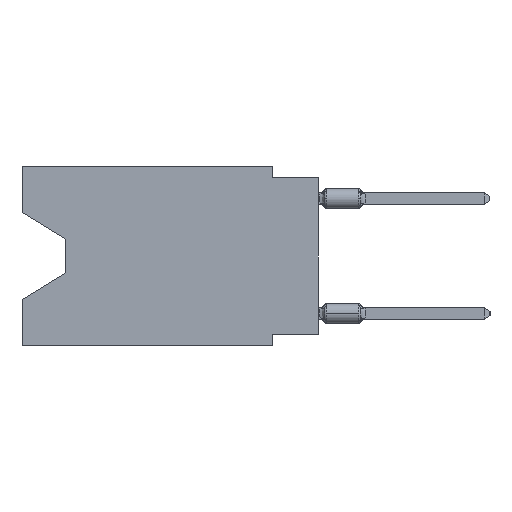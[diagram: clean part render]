
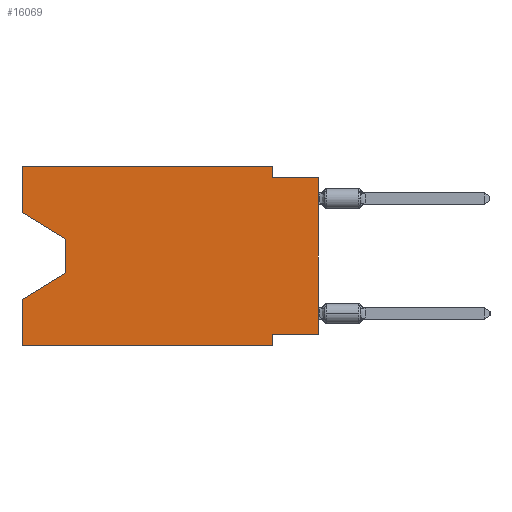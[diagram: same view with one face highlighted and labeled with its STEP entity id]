
A CAD part, left-side view. The second image highlights one B-rep face of the part: STEP entity #16069.
In plain terms, the highlighted planar face has unit normal (-1, 0, 0).
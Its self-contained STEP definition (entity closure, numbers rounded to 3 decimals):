
#253 = DIRECTION ( 'NONE',  ( 0., -0.855, -0.519 ) ) ;
#407 = VECTOR ( 'NONE', #17483, 1000. ) ;
#1360 = CARTESIAN_POINT ( 'NONE',  ( 0., 0., -9.271 ) ) ;
#1849 = LINE ( 'NONE', #1360, #12850 ) ;
#1931 = LINE ( 'NONE', #11982, #15742 ) ;
#2307 = LINE ( 'NONE', #31834, #407 ) ;
#2446 = EDGE_CURVE ( 'NONE', #3500, #23172, #26357, .T. ) ;
#2697 = ORIENTED_EDGE ( 'NONE', *, *, #17128, .T. ) ;
#2833 = ORIENTED_EDGE ( 'NONE', *, *, #22995, .F. ) ;
#3056 = CARTESIAN_POINT ( 'NONE',  ( 0., 16.383, -2.546 ) ) ;
#3317 = VECTOR ( 'NONE', #18878, 1000. ) ;
#3348 = EDGE_CURVE ( 'NONE', #29747, #30917, #1849, .T. ) ;
#3500 = VERTEX_POINT ( 'NONE', #32190 ) ;
#4700 = ORIENTED_EDGE ( 'NONE', *, *, #19175, .F. ) ;
#5203 = CARTESIAN_POINT ( 'NONE',  ( 0., 16.383, -9.906 ) ) ;
#6359 = VERTEX_POINT ( 'NONE', #16911 ) ;
#6776 = CARTESIAN_POINT ( 'NONE',  ( 0., 2.54, -9.271 ) ) ;
#7807 = LINE ( 'NONE', #28116, #12186 ) ;
#7935 = VECTOR ( 'NONE', #253, 1000. ) ;
#8007 = VERTEX_POINT ( 'NONE', #12410 ) ;
#8150 = LINE ( 'NONE', #10787, #27226 ) ;
#8793 = CARTESIAN_POINT ( 'NONE',  ( 0., 13.97, -5.893 ) ) ;
#9356 = VERTEX_POINT ( 'NONE', #8793 ) ;
#9927 = CARTESIAN_POINT ( 'NONE',  ( 0., 2.54, -9.906 ) ) ;
#10622 = EDGE_CURVE ( 'NONE', #30917, #29506, #10952, .T. ) ;
#10629 = LINE ( 'NONE', #3056, #7935 ) ;
#10787 = CARTESIAN_POINT ( 'NONE',  ( 0., 16.383, 0. ) ) ;
#10952 = LINE ( 'NONE', #31084, #3317 ) ;
#11600 = ORIENTED_EDGE ( 'NONE', *, *, #25312, .T. ) ;
#11870 = ORIENTED_EDGE ( 'NONE', *, *, #10622, .F. ) ;
#11897 = DIRECTION ( 'NONE',  ( 0., 1., 0. ) ) ;
#11982 = CARTESIAN_POINT ( 'NONE',  ( 0., 13.97, -5.893 ) ) ;
#12186 = VECTOR ( 'NONE', #30104, 1000. ) ;
#12410 = CARTESIAN_POINT ( 'NONE',  ( 0., 16.383, -2.546 ) ) ;
#12850 = VECTOR ( 'NONE', #11897, 1000. ) ;
#13371 = ORIENTED_EDGE ( 'NONE', *, *, #19501, .T. ) ;
#13765 = VECTOR ( 'NONE', #29118, 1000. ) ;
#13810 = CARTESIAN_POINT ( 'NONE',  ( 0., 16.383, 0. ) ) ;
#14072 = AXIS2_PLACEMENT_3D ( 'NONE', #29518, #21774, #19460 ) ;
#14195 = CARTESIAN_POINT ( 'NONE',  ( 0., 0., -9.271 ) ) ;
#14386 = LINE ( 'NONE', #31880, #29523 ) ;
#14493 = FACE_OUTER_BOUND ( 'NONE', #32248, .T. ) ;
#15328 = ORIENTED_EDGE ( 'NONE', *, *, #3348, .F. ) ;
#15532 = EDGE_CURVE ( 'NONE', #20619, #28723, #8150, .T. ) ;
#15742 = VECTOR ( 'NONE', #22058, 1000. ) ;
#15854 = ORIENTED_EDGE ( 'NONE', *, *, #15532, .F. ) ;
#16069 = ADVANCED_FACE ( 'NONE', ( #14493 ), #27216, .F. ) ;
#16404 = EDGE_CURVE ( 'NONE', #23172, #27235, #29970, .T. ) ;
#16911 = CARTESIAN_POINT ( 'NONE',  ( 0., 0., -0.635 ) ) ;
#17128 = EDGE_CURVE ( 'NONE', #20619, #29506, #18854, .T. ) ;
#17483 = DIRECTION ( 'NONE',  ( 0., 0., 1. ) ) ;
#18854 = LINE ( 'NONE', #28923, #22419 ) ;
#18878 = DIRECTION ( 'NONE',  ( 0., 0., -1. ) ) ;
#19046 = LINE ( 'NONE', #21842, #13765 ) ;
#19081 = VECTOR ( 'NONE', #28669, 1000. ) ;
#19175 = EDGE_CURVE ( 'NONE', #27235, #6359, #7807, .T. ) ;
#19460 = DIRECTION ( 'NONE',  ( 0., 0., -1. ) ) ;
#19501 = EDGE_CURVE ( 'NONE', #28805, #9356, #14386, .T. ) ;
#20581 = EDGE_CURVE ( 'NONE', #8007, #28805, #10629, .T. ) ;
#20619 = VERTEX_POINT ( 'NONE', #5203 ) ;
#20765 = EDGE_CURVE ( 'NONE', #29747, #6359, #19046, .T. ) ;
#21084 = CARTESIAN_POINT ( 'NONE',  ( 0., 2.54, 0. ) ) ;
#21774 = DIRECTION ( 'NONE',  ( 1., 0., 0. ) ) ;
#21842 = CARTESIAN_POINT ( 'NONE',  ( 0., 0., 0. ) ) ;
#22058 = DIRECTION ( 'NONE',  ( 0., 0.855, -0.519 ) ) ;
#22383 = DIRECTION ( 'NONE',  ( 0., 0., -1. ) ) ;
#22419 = VECTOR ( 'NONE', #25541, 1000. ) ;
#22552 = CARTESIAN_POINT ( 'NONE',  ( 0., 2.54, 0. ) ) ;
#22915 = CARTESIAN_POINT ( 'NONE',  ( 0., 13.97, -4.013 ) ) ;
#22995 = EDGE_CURVE ( 'NONE', #8007, #3500, #2307, .T. ) ;
#23172 = VERTEX_POINT ( 'NONE', #21084 ) ;
#23569 = VECTOR ( 'NONE', #22383, 1000. ) ;
#23577 = CARTESIAN_POINT ( 'NONE',  ( 0., 16.383, -7.36 ) ) ;
#24458 = DIRECTION ( 'NONE',  ( 0., 0., -1. ) ) ;
#24817 = ORIENTED_EDGE ( 'NONE', *, *, #16404, .F. ) ;
#25312 = EDGE_CURVE ( 'NONE', #9356, #28723, #1931, .T. ) ;
#25541 = DIRECTION ( 'NONE',  ( 0., -1., 0. ) ) ;
#26290 = CARTESIAN_POINT ( 'NONE',  ( 0., 2.54, -0.635 ) ) ;
#26357 = LINE ( 'NONE', #13810, #19081 ) ;
#27216 = PLANE ( 'NONE',  #14072 ) ;
#27226 = VECTOR ( 'NONE', #28796, 1000. ) ;
#27235 = VERTEX_POINT ( 'NONE', #26290 ) ;
#27630 = ORIENTED_EDGE ( 'NONE', *, *, #20581, .T. ) ;
#28116 = CARTESIAN_POINT ( 'NONE',  ( 0., 0., -0.635 ) ) ;
#28669 = DIRECTION ( 'NONE',  ( 0., -1., 0. ) ) ;
#28723 = VERTEX_POINT ( 'NONE', #23577 ) ;
#28760 = ORIENTED_EDGE ( 'NONE', *, *, #2446, .F. ) ;
#28796 = DIRECTION ( 'NONE',  ( 0., 0., 1. ) ) ;
#28805 = VERTEX_POINT ( 'NONE', #22915 ) ;
#28923 = CARTESIAN_POINT ( 'NONE',  ( 0., 16.383, -9.906 ) ) ;
#29118 = DIRECTION ( 'NONE',  ( 0., 0., 1. ) ) ;
#29506 = VERTEX_POINT ( 'NONE', #9927 ) ;
#29518 = CARTESIAN_POINT ( 'NONE',  ( 0., 16.383, 0. ) ) ;
#29523 = VECTOR ( 'NONE', #24458, 1000. ) ;
#29747 = VERTEX_POINT ( 'NONE', #14195 ) ;
#29970 = LINE ( 'NONE', #22552, #23569 ) ;
#30104 = DIRECTION ( 'NONE',  ( 0., -1., 0. ) ) ;
#30917 = VERTEX_POINT ( 'NONE', #6776 ) ;
#31084 = CARTESIAN_POINT ( 'NONE',  ( 0., 2.54, -9.906 ) ) ;
#31834 = CARTESIAN_POINT ( 'NONE',  ( 0., 16.383, 0. ) ) ;
#31880 = CARTESIAN_POINT ( 'NONE',  ( 0., 13.97, -4.013 ) ) ;
#32061 = ORIENTED_EDGE ( 'NONE', *, *, #20765, .T. ) ;
#32190 = CARTESIAN_POINT ( 'NONE',  ( 0., 16.383, 0. ) ) ;
#32248 = EDGE_LOOP ( 'NONE', ( #27630, #13371, #11600, #15854, #2697, #11870, #15328, #32061, #4700, #24817, #28760, #2833 ) ) ;
